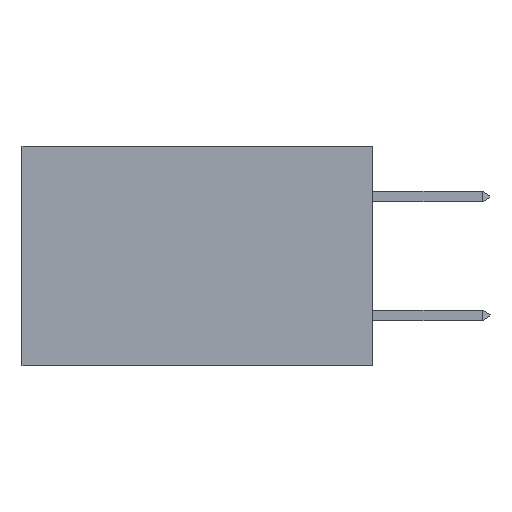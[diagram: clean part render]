
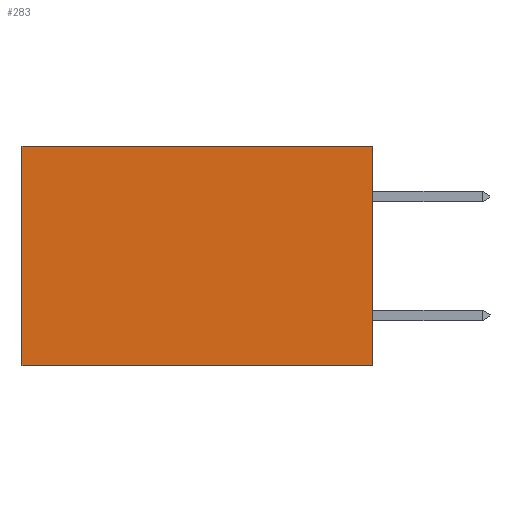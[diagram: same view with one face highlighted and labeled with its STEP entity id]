
A CAD part, left-side view. The second image highlights one B-rep face of the part: STEP entity #283.
In plain terms, the highlighted planar face has unit normal (-1, 0, 0).
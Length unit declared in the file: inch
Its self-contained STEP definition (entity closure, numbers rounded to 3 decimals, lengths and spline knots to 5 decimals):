
#283 = ADVANCED_FACE ( 'NONE', ( #8743 ), #927, .F. ) ;
#927 = PLANE ( 'NONE',  #6708 ) ;
#2160 = EDGE_CURVE ( 'NONE', #7624, #11092, #18370, .T. ) ;
#2660 = VECTOR ( 'NONE', #13139, 39.37008 ) ;
#3411 = VECTOR ( 'NONE', #5335, 39.37008 ) ;
#3528 = ORIENTED_EDGE ( 'NONE', *, *, #5045, .T. ) ;
#4552 = VECTOR ( 'NONE', #18583, 39.37008 ) ;
#5045 = EDGE_CURVE ( 'NONE', #19166, #11555, #20093, .T. ) ;
#5335 = DIRECTION ( 'NONE',  ( 0., 0., -1. ) ) ;
#5367 = CARTESIAN_POINT ( 'NONE',  ( 0.277, 0.59, 0. ) ) ;
#5406 = CARTESIAN_POINT ( 'NONE',  ( 0.277, 0., 0. ) ) ;
#6653 = ORIENTED_EDGE ( 'NONE', *, *, #2160, .F. ) ;
#6708 = AXIS2_PLACEMENT_3D ( 'NONE', #8676, #8920, #8914 ) ;
#7624 = VERTEX_POINT ( 'NONE', #5406 ) ;
#8676 = CARTESIAN_POINT ( 'NONE',  ( 0.277, 0., -0.37 ) ) ;
#8743 = FACE_OUTER_BOUND ( 'NONE', #17403, .T. ) ;
#8747 = CARTESIAN_POINT ( 'NONE',  ( 0.277, 0., -0.37 ) ) ;
#8914 = DIRECTION ( 'NONE',  ( 0., 0., -1. ) ) ;
#8920 = DIRECTION ( 'NONE',  ( 1., 0., 0. ) ) ;
#9251 = CARTESIAN_POINT ( 'NONE',  ( 0.277, 0., -0.37 ) ) ;
#9429 = VECTOR ( 'NONE', #10375, 39.37008 ) ;
#10375 = DIRECTION ( 'NONE',  ( 0., 1., 0. ) ) ;
#10971 = EDGE_CURVE ( 'NONE', #7624, #19166, #24271, .T. ) ;
#11092 = VERTEX_POINT ( 'NONE', #8747 ) ;
#11271 = EDGE_CURVE ( 'NONE', #11092, #11555, #17625, .T. ) ;
#11555 = VERTEX_POINT ( 'NONE', #19776 ) ;
#13139 = DIRECTION ( 'NONE',  ( 0., 1., 0. ) ) ;
#17034 = ORIENTED_EDGE ( 'NONE', *, *, #11271, .F. ) ;
#17403 = EDGE_LOOP ( 'NONE', ( #3528, #17034, #6653, #19237 ) ) ;
#17625 = LINE ( 'NONE', #9251, #2660 ) ;
#17956 = CARTESIAN_POINT ( 'NONE',  ( 0.277, 0., -0.37 ) ) ;
#18370 = LINE ( 'NONE', #17956, #3411 ) ;
#18583 = DIRECTION ( 'NONE',  ( 0., 0., -1. ) ) ;
#18836 = CARTESIAN_POINT ( 'NONE',  ( 0.277, 0.59, -0.37 ) ) ;
#19166 = VERTEX_POINT ( 'NONE', #5367 ) ;
#19237 = ORIENTED_EDGE ( 'NONE', *, *, #10971, .T. ) ;
#19776 = CARTESIAN_POINT ( 'NONE',  ( 0.277, 0.59, -0.37 ) ) ;
#20093 = LINE ( 'NONE', #18836, #4552 ) ;
#22006 = CARTESIAN_POINT ( 'NONE',  ( 0.277, 0., 0. ) ) ;
#24271 = LINE ( 'NONE', #22006, #9429 ) ;
